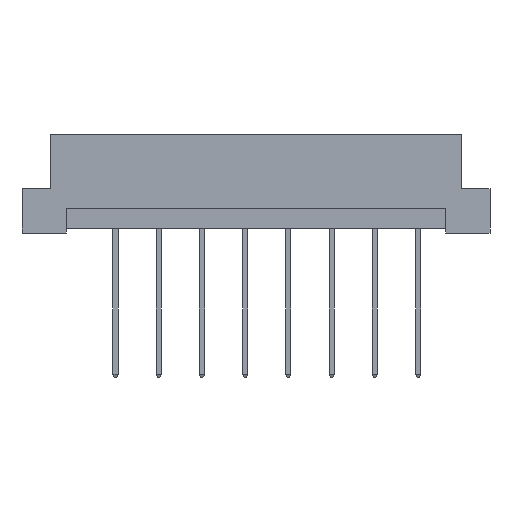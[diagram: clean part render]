
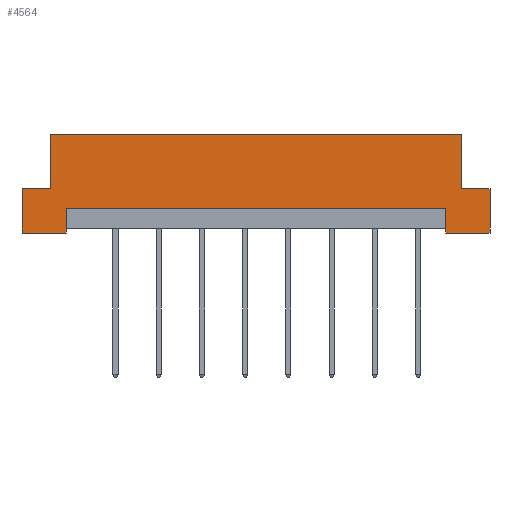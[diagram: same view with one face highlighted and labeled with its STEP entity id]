
A CAD part, front view. The second image highlights one B-rep face of the part: STEP entity #4564.
In plain terms, the highlighted planar face has unit normal (0, -1, 0).
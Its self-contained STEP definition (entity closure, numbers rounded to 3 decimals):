
#42 = VECTOR ( 'NONE', #4812, 1000. ) ;
#137 = VECTOR ( 'NONE', #5165, 1000. ) ;
#140 = CARTESIAN_POINT ( 'NONE',  ( 27.5, 0., 0. ) ) ;
#393 = CARTESIAN_POINT ( 'NONE',  ( 22.3, 0., 0. ) ) ;
#398 = CARTESIAN_POINT ( 'NONE',  ( 24.2, 0., 5.2 ) ) ;
#453 = EDGE_CURVE ( 'NONE', #5901, #1055, #6497, .T. ) ;
#518 = CARTESIAN_POINT ( 'NONE',  ( -27.5, 0., 11.6 ) ) ;
#796 = CARTESIAN_POINT ( 'NONE',  ( -27.5, 0., 0. ) ) ;
#820 = CARTESIAN_POINT ( 'NONE',  ( -27.5, 0., 0. ) ) ;
#1055 = VERTEX_POINT ( 'NONE', #393 ) ;
#1223 = LINE ( 'NONE', #6862, #7231 ) ;
#1641 = PLANE ( 'NONE',  #2218 ) ;
#1644 = CARTESIAN_POINT ( 'NONE',  ( 22.3, 0., 2.9 ) ) ;
#1680 = EDGE_CURVE ( 'NONE', #8648, #2195, #6795, .T. ) ;
#1687 = CARTESIAN_POINT ( 'NONE',  ( -27.5, 0., 11.6 ) ) ;
#1713 = DIRECTION ( 'NONE',  ( -1., 0., 0. ) ) ;
#1757 = EDGE_CURVE ( 'NONE', #6729, #5060, #8581, .T. ) ;
#1798 = LINE ( 'NONE', #6696, #7631 ) ;
#1802 = VERTEX_POINT ( 'NONE', #3569 ) ;
#1949 = DIRECTION ( 'NONE',  ( -1., 0., 0. ) ) ;
#2012 = ORIENTED_EDGE ( 'NONE', *, *, #1680, .F. ) ;
#2156 = VERTEX_POINT ( 'NONE', #140 ) ;
#2195 = VERTEX_POINT ( 'NONE', #4848 ) ;
#2218 = AXIS2_PLACEMENT_3D ( 'NONE', #1687, #2958, #4426 ) ;
#2365 = ORIENTED_EDGE ( 'NONE', *, *, #3693, .F. ) ;
#2454 = LINE ( 'NONE', #398, #4543 ) ;
#2458 = ORIENTED_EDGE ( 'NONE', *, *, #3870, .F. ) ;
#2898 = EDGE_CURVE ( 'NONE', #5039, #6729, #3561, .T. ) ;
#2934 = ORIENTED_EDGE ( 'NONE', *, *, #5375, .F. ) ;
#2958 = DIRECTION ( 'NONE',  ( 0., 1., 0. ) ) ;
#3250 = ORIENTED_EDGE ( 'NONE', *, *, #6620, .F. ) ;
#3278 = DIRECTION ( 'NONE',  ( 0., 0., 1. ) ) ;
#3363 = ORIENTED_EDGE ( 'NONE', *, *, #453, .T. ) ;
#3424 = VECTOR ( 'NONE', #3503, 1000. ) ;
#3503 = DIRECTION ( 'NONE',  ( -1., 0., 0. ) ) ;
#3540 = CARTESIAN_POINT ( 'NONE',  ( 24.2, 0., 5.2 ) ) ;
#3561 = LINE ( 'NONE', #820, #137 ) ;
#3569 = CARTESIAN_POINT ( 'NONE',  ( -22.3, 0., 0. ) ) ;
#3693 = EDGE_CURVE ( 'NONE', #2156, #1055, #4740, .T. ) ;
#3766 = CARTESIAN_POINT ( 'NONE',  ( -22.3, 0., 2.9 ) ) ;
#3870 = EDGE_CURVE ( 'NONE', #4422, #2156, #8858, .T. ) ;
#4077 = EDGE_LOOP ( 'NONE', ( #4635, #3363, #2365, #2458, #2934, #5114, #2012, #6086, #7313, #6451, #8592, #3250 ) ) ;
#4104 = VECTOR ( 'NONE', #7576, 1000. ) ;
#4139 = LINE ( 'NONE', #6389, #3424 ) ;
#4228 = CARTESIAN_POINT ( 'NONE',  ( -24.2, 0., 5.2 ) ) ;
#4422 = VERTEX_POINT ( 'NONE', #7738 ) ;
#4426 = DIRECTION ( 'NONE',  ( 0., 0., 1. ) ) ;
#4463 = LINE ( 'NONE', #7170, #8995 ) ;
#4543 = VECTOR ( 'NONE', #3278, 1000. ) ;
#4564 = ADVANCED_FACE ( 'NONE', ( #6447 ), #1641, .F. ) ;
#4635 = ORIENTED_EDGE ( 'NONE', *, *, #5594, .F. ) ;
#4740 = LINE ( 'NONE', #6203, #7574 ) ;
#4772 = CARTESIAN_POINT ( 'NONE',  ( 27.5, 0., 5.2 ) ) ;
#4812 = DIRECTION ( 'NONE',  ( 1., 0., 0. ) ) ;
#4819 = EDGE_CURVE ( 'NONE', #5075, #2195, #2454, .T. ) ;
#4848 = CARTESIAN_POINT ( 'NONE',  ( 24.2, 0., 11.6 ) ) ;
#4993 = DIRECTION ( 'NONE',  ( 1., 0., 0. ) ) ;
#5039 = VERTEX_POINT ( 'NONE', #796 ) ;
#5060 = VERTEX_POINT ( 'NONE', #4228 ) ;
#5075 = VERTEX_POINT ( 'NONE', #3540 ) ;
#5114 = ORIENTED_EDGE ( 'NONE', *, *, #4819, .T. ) ;
#5160 = DIRECTION ( 'NONE',  ( 0., 0., -1. ) ) ;
#5165 = DIRECTION ( 'NONE',  ( 0., 0., 1. ) ) ;
#5271 = DIRECTION ( 'NONE',  ( 0., 0., -1. ) ) ;
#5375 = EDGE_CURVE ( 'NONE', #5075, #4422, #9050, .T. ) ;
#5594 = EDGE_CURVE ( 'NONE', #5901, #6201, #1798, .T. ) ;
#5649 = DIRECTION ( 'NONE',  ( 0., 0., 1. ) ) ;
#5681 = CARTESIAN_POINT ( 'NONE',  ( -27.5, 0., 5.2 ) ) ;
#5901 = VERTEX_POINT ( 'NONE', #1644 ) ;
#6086 = ORIENTED_EDGE ( 'NONE', *, *, #6281, .F. ) ;
#6201 = VERTEX_POINT ( 'NONE', #3766 ) ;
#6203 = CARTESIAN_POINT ( 'NONE',  ( -27.5, 0., 0. ) ) ;
#6210 = CARTESIAN_POINT ( 'NONE',  ( -27.5, 0., 5.2 ) ) ;
#6281 = EDGE_CURVE ( 'NONE', #5060, #8648, #4463, .T. ) ;
#6389 = CARTESIAN_POINT ( 'NONE',  ( -27.5, 0., 0. ) ) ;
#6447 = FACE_OUTER_BOUND ( 'NONE', #4077, .T. ) ;
#6451 = ORIENTED_EDGE ( 'NONE', *, *, #2898, .F. ) ;
#6453 = CARTESIAN_POINT ( 'NONE',  ( 22.3, 0., 0.5 ) ) ;
#6497 = LINE ( 'NONE', #6453, #8630 ) ;
#6620 = EDGE_CURVE ( 'NONE', #6201, #1802, #1223, .T. ) ;
#6696 = CARTESIAN_POINT ( 'NONE',  ( 22.3, 0., 2.9 ) ) ;
#6729 = VERTEX_POINT ( 'NONE', #6210 ) ;
#6745 = CARTESIAN_POINT ( 'NONE',  ( 27.5, 0., 0. ) ) ;
#6750 = EDGE_CURVE ( 'NONE', #1802, #5039, #4139, .T. ) ;
#6770 = DIRECTION ( 'NONE',  ( 0., 0., -1. ) ) ;
#6795 = LINE ( 'NONE', #518, #42 ) ;
#6862 = CARTESIAN_POINT ( 'NONE',  ( -22.3, 0., 0.5 ) ) ;
#7170 = CARTESIAN_POINT ( 'NONE',  ( -24.2, 0., 5.2 ) ) ;
#7231 = VECTOR ( 'NONE', #6770, 1000. ) ;
#7313 = ORIENTED_EDGE ( 'NONE', *, *, #1757, .F. ) ;
#7348 = CARTESIAN_POINT ( 'NONE',  ( -24.2, 0., 11.6 ) ) ;
#7574 = VECTOR ( 'NONE', #1949, 1000. ) ;
#7576 = DIRECTION ( 'NONE',  ( 1., 0., 0. ) ) ;
#7631 = VECTOR ( 'NONE', #1713, 1000. ) ;
#7738 = CARTESIAN_POINT ( 'NONE',  ( 27.5, 0., 5.2 ) ) ;
#7858 = VECTOR ( 'NONE', #4993, 1000. ) ;
#7872 = VECTOR ( 'NONE', #5271, 1000. ) ;
#8581 = LINE ( 'NONE', #5681, #7858 ) ;
#8592 = ORIENTED_EDGE ( 'NONE', *, *, #6750, .F. ) ;
#8630 = VECTOR ( 'NONE', #5160, 1000. ) ;
#8648 = VERTEX_POINT ( 'NONE', #7348 ) ;
#8858 = LINE ( 'NONE', #6745, #7872 ) ;
#8995 = VECTOR ( 'NONE', #5649, 1000. ) ;
#9050 = LINE ( 'NONE', #4772, #4104 ) ;
